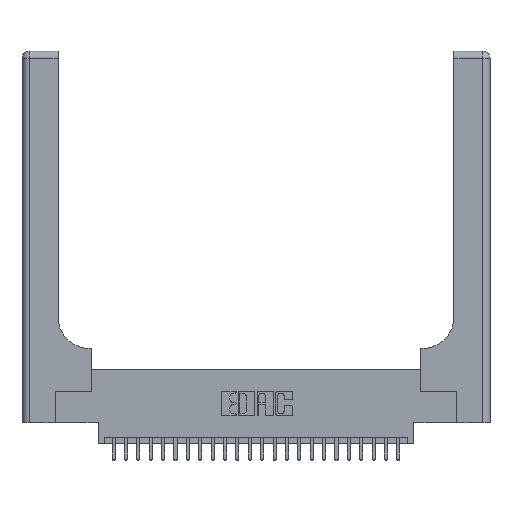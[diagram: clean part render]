
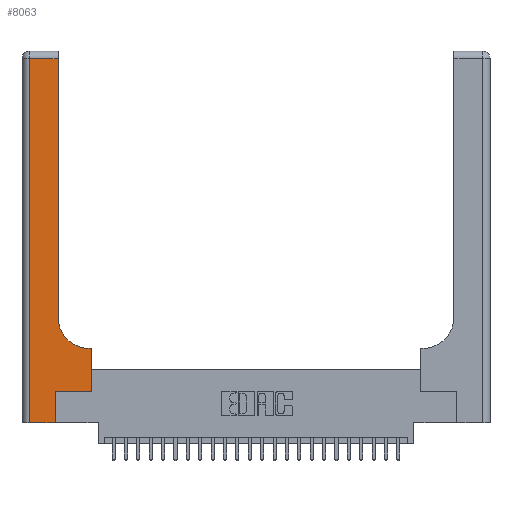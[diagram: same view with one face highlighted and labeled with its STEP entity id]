
A CAD part, top view. The second image highlights one B-rep face of the part: STEP entity #8063.
In plain terms, the highlighted planar face has unit normal (0, 0, 1).
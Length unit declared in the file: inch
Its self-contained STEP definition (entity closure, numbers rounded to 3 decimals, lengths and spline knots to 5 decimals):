
#256 = EDGE_CURVE ( 'NONE', #13471, #22514, #25436, .T. ) ;
#459 = LINE ( 'NONE', #17320, #15764 ) ;
#515 = DIRECTION ( 'NONE',  ( 0., -1., 0. ) ) ;
#613 = CARTESIAN_POINT ( 'NONE',  ( 0.06, 3., 0.37 ) ) ;
#1342 = VERTEX_POINT ( 'NONE', #6952 ) ;
#1659 = EDGE_CURVE ( 'NONE', #14313, #20685, #6278, .T. ) ;
#1953 = DIRECTION ( 'NONE',  ( 0., 1., 0. ) ) ;
#3175 = CARTESIAN_POINT ( 'NONE',  ( 0., 0., 0.37 ) ) ;
#3367 = LINE ( 'NONE', #25296, #25093 ) ;
#3528 = CARTESIAN_POINT ( 'NONE',  ( 0., 3., 0.37 ) ) ;
#4653 = EDGE_CURVE ( 'NONE', #20281, #6245, #26499, .T. ) ;
#4770 = CARTESIAN_POINT ( 'NONE',  ( 0.269, 0.25, 0.37 ) ) ;
#4896 = VERTEX_POINT ( 'NONE', #20198 ) ;
#5322 = LINE ( 'NONE', #3175, #16283 ) ;
#5605 = PLANE ( 'NONE',  #13086 ) ;
#5698 = CARTESIAN_POINT ( 'NONE',  ( 0.5585, 0.25, 0.37 ) ) ;
#6006 = CARTESIAN_POINT ( 'NONE',  ( 0.5415, 0.6, 0.37 ) ) ;
#6245 = VERTEX_POINT ( 'NONE', #5698 ) ;
#6278 = LINE ( 'NONE', #613, #16591 ) ;
#6618 = ORIENTED_EDGE ( 'NONE', *, *, #21815, .T. ) ;
#6952 = CARTESIAN_POINT ( 'NONE',  ( 0.2915, 2.94, 0.37 ) ) ;
#7253 = DIRECTION ( 'NONE',  ( 1., 0., 0. ) ) ;
#7695 = DIRECTION ( 'NONE',  ( 0., 0., -1. ) ) ;
#7973 = VERTEX_POINT ( 'NONE', #23757 ) ;
#8063 = ADVANCED_FACE ( 'NONE', ( #25902 ), #5605, .F. ) ;
#8601 = ORIENTED_EDGE ( 'NONE', *, *, #20210, .T. ) ;
#8803 = DIRECTION ( 'NONE',  ( -1., 0., 0. ) ) ;
#9253 = ORIENTED_EDGE ( 'NONE', *, *, #256, .T. ) ;
#10056 = CARTESIAN_POINT ( 'NONE',  ( 0.06, 0., 0.37 ) ) ;
#10904 = EDGE_LOOP ( 'NONE', ( #16927, #6618, #12776, #18202, #13440, #24214, #8601, #24824, #9253 ) ) ;
#11134 = LINE ( 'NONE', #21606, #15940 ) ;
#11519 = EDGE_CURVE ( 'NONE', #20685, #7973, #5322, .T. ) ;
#12204 = EDGE_CURVE ( 'NONE', #22514, #1342, #11134, .T. ) ;
#12309 = CARTESIAN_POINT ( 'NONE',  ( 0.5585, 0.25, 0.37 ) ) ;
#12743 = CARTESIAN_POINT ( 'NONE',  ( 0.06, 2.94, 0.37 ) ) ;
#12776 = ORIENTED_EDGE ( 'NONE', *, *, #1659, .T. ) ;
#13086 = AXIS2_PLACEMENT_3D ( 'NONE', #3528, #7695, #21983 ) ;
#13190 = DIRECTION ( 'NONE',  ( 0., 1., 0. ) ) ;
#13440 = ORIENTED_EDGE ( 'NONE', *, *, #20481, .T. ) ;
#13471 = VERTEX_POINT ( 'NONE', #6006 ) ;
#13548 = DIRECTION ( 'NONE',  ( 0., 1., 0. ) ) ;
#14313 = VERTEX_POINT ( 'NONE', #12743 ) ;
#14545 = CARTESIAN_POINT ( 'NONE',  ( 0.269, 0.25, 0.37 ) ) ;
#15565 = VECTOR ( 'NONE', #8803, 39.37008 ) ;
#15764 = VECTOR ( 'NONE', #21368, 39.37008 ) ;
#15940 = VECTOR ( 'NONE', #13548, 39.37008 ) ;
#16283 = VECTOR ( 'NONE', #7253, 39.37008 ) ;
#16591 = VECTOR ( 'NONE', #515, 39.37008 ) ;
#16927 = ORIENTED_EDGE ( 'NONE', *, *, #12204, .T. ) ;
#17114 = DIRECTION ( 'NONE',  ( 1., 0., 0. ) ) ;
#17320 = CARTESIAN_POINT ( 'NONE',  ( 0.2915, 0.6, 0.37 ) ) ;
#18202 = ORIENTED_EDGE ( 'NONE', *, *, #11519, .T. ) ;
#18969 = CARTESIAN_POINT ( 'NONE',  ( 0., 2.94, 0.37 ) ) ;
#19928 = EDGE_CURVE ( 'NONE', #4896, #13471, #459, .T. ) ;
#20170 = LINE ( 'NONE', #12309, #20785 ) ;
#20198 = CARTESIAN_POINT ( 'NONE',  ( 0.5585, 0.6, 0.37 ) ) ;
#20210 = EDGE_CURVE ( 'NONE', #6245, #4896, #20170, .T. ) ;
#20281 = VERTEX_POINT ( 'NONE', #14545 ) ;
#20481 = EDGE_CURVE ( 'NONE', #7973, #20281, #3367, .T. ) ;
#20685 = VERTEX_POINT ( 'NONE', #10056 ) ;
#20785 = VECTOR ( 'NONE', #1953, 39.37008 ) ;
#21164 = VECTOR ( 'NONE', #17114, 39.37008 ) ;
#21368 = DIRECTION ( 'NONE',  ( -1., 0., 0. ) ) ;
#21478 = AXIS2_PLACEMENT_3D ( 'NONE', #26126, #26095, #26072 ) ;
#21567 = LINE ( 'NONE', #18969, #15565 ) ;
#21606 = CARTESIAN_POINT ( 'NONE',  ( 0.2915, 3., 0.37 ) ) ;
#21815 = EDGE_CURVE ( 'NONE', #1342, #14313, #21567, .T. ) ;
#21983 = DIRECTION ( 'NONE',  ( -1., 0., 0. ) ) ;
#22514 = VERTEX_POINT ( 'NONE', #25380 ) ;
#23757 = CARTESIAN_POINT ( 'NONE',  ( 0.269, 0., 0.37 ) ) ;
#24214 = ORIENTED_EDGE ( 'NONE', *, *, #4653, .T. ) ;
#24824 = ORIENTED_EDGE ( 'NONE', *, *, #19928, .T. ) ;
#25093 = VECTOR ( 'NONE', #13190, 39.37008 ) ;
#25296 = CARTESIAN_POINT ( 'NONE',  ( 0.269, 0., 0.37 ) ) ;
#25380 = CARTESIAN_POINT ( 'NONE',  ( 0.2915, 0.85, 0.37 ) ) ;
#25436 = CIRCLE ( 'NONE', #21478, 0.25 ) ;
#25902 = FACE_OUTER_BOUND ( 'NONE', #10904, .T. ) ;
#26072 = DIRECTION ( 'NONE',  ( 1., 0., 0. ) ) ;
#26095 = DIRECTION ( 'NONE',  ( 0., 0., -1. ) ) ;
#26126 = CARTESIAN_POINT ( 'NONE',  ( 0.5415, 0.85, 0.37 ) ) ;
#26499 = LINE ( 'NONE', #4770, #21164 ) ;
